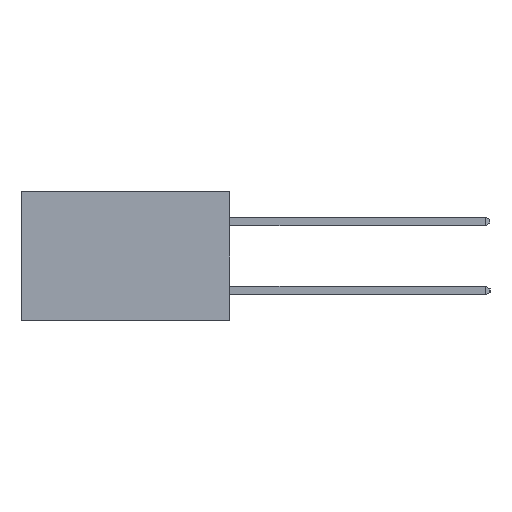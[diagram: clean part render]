
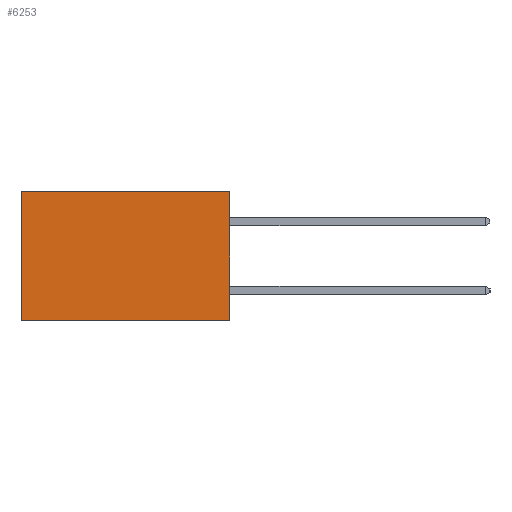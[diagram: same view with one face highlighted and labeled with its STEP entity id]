
A CAD part, left-side view. The second image highlights one B-rep face of the part: STEP entity #6253.
In plain terms, the highlighted planar face has unit normal (-1, 0, 0).
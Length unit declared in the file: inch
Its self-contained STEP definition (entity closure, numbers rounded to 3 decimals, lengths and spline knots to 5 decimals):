
#1555 = CARTESIAN_POINT ( 'NONE',  ( 0.2615, 0.6, -0.37 ) ) ;
#3198 = DIRECTION ( 'NONE',  ( 0., 0., -1. ) ) ;
#3415 = DIRECTION ( 'NONE',  ( 1., 0., 0. ) ) ;
#3652 = CARTESIAN_POINT ( 'NONE',  ( 0.2615, 0., -0.37 ) ) ;
#4817 = DIRECTION ( 'NONE',  ( 0., 0., -1. ) ) ;
#5011 = PLANE ( 'NONE',  #21493 ) ;
#5131 = VERTEX_POINT ( 'NONE', #11785 ) ;
#5522 = VERTEX_POINT ( 'NONE', #1555 ) ;
#5870 = LINE ( 'NONE', #15278, #19661 ) ;
#6253 = ADVANCED_FACE ( 'NONE', ( #14812 ), #5011, .F. ) ;
#6565 = EDGE_CURVE ( 'NONE', #5131, #5522, #22798, .T. ) ;
#8568 = CARTESIAN_POINT ( 'NONE',  ( 0.2615, 0., -0.37 ) ) ;
#8719 = VERTEX_POINT ( 'NONE', #8907 ) ;
#8907 = CARTESIAN_POINT ( 'NONE',  ( 0.2615, 0., -0.37 ) ) ;
#9842 = DIRECTION ( 'NONE',  ( 0., 1., 0. ) ) ;
#10016 = LINE ( 'NONE', #8568, #14806 ) ;
#10391 = ORIENTED_EDGE ( 'NONE', *, *, #13816, .F. ) ;
#10787 = VERTEX_POINT ( 'NONE', #20826 ) ;
#10858 = EDGE_CURVE ( 'NONE', #10787, #8719, #10016, .T. ) ;
#11785 = CARTESIAN_POINT ( 'NONE',  ( 0.2615, 0.6, 0. ) ) ;
#11951 = ORIENTED_EDGE ( 'NONE', *, *, #6565, .T. ) ;
#13816 = EDGE_CURVE ( 'NONE', #8719, #5522, #5870, .T. ) ;
#14806 = VECTOR ( 'NONE', #4817, 39.37008 ) ;
#14812 = FACE_OUTER_BOUND ( 'NONE', #17836, .T. ) ;
#15278 = CARTESIAN_POINT ( 'NONE',  ( 0.2615, 0., -0.37 ) ) ;
#16526 = CARTESIAN_POINT ( 'NONE',  ( 0.2615, 0.6, -0.37 ) ) ;
#17019 = VECTOR ( 'NONE', #23107, 39.37008 ) ;
#17836 = EDGE_LOOP ( 'NONE', ( #11951, #10391, #22943, #20453 ) ) ;
#19661 = VECTOR ( 'NONE', #9842, 39.37008 ) ;
#20329 = CARTESIAN_POINT ( 'NONE',  ( 0.2615, 0., 0. ) ) ;
#20453 = ORIENTED_EDGE ( 'NONE', *, *, #21068, .T. ) ;
#20826 = CARTESIAN_POINT ( 'NONE',  ( 0.2615, 0., 0. ) ) ;
#21068 = EDGE_CURVE ( 'NONE', #10787, #5131, #23279, .T. ) ;
#21493 = AXIS2_PLACEMENT_3D ( 'NONE', #3652, #3415, #3198 ) ;
#22096 = DIRECTION ( 'NONE',  ( 0., 1., 0. ) ) ;
#22730 = VECTOR ( 'NONE', #22096, 39.37008 ) ;
#22798 = LINE ( 'NONE', #16526, #17019 ) ;
#22943 = ORIENTED_EDGE ( 'NONE', *, *, #10858, .F. ) ;
#23107 = DIRECTION ( 'NONE',  ( 0., 0., -1. ) ) ;
#23279 = LINE ( 'NONE', #20329, #22730 ) ;
